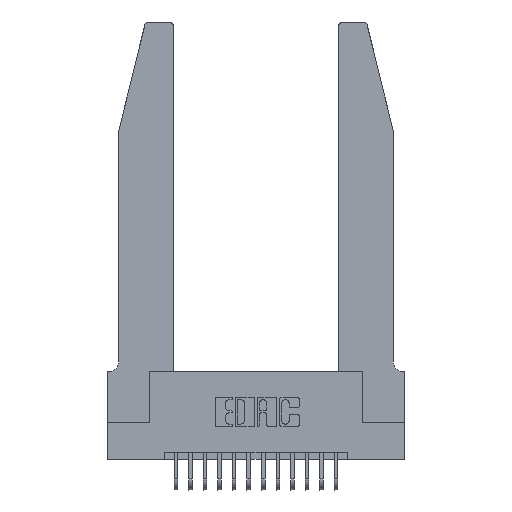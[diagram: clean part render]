
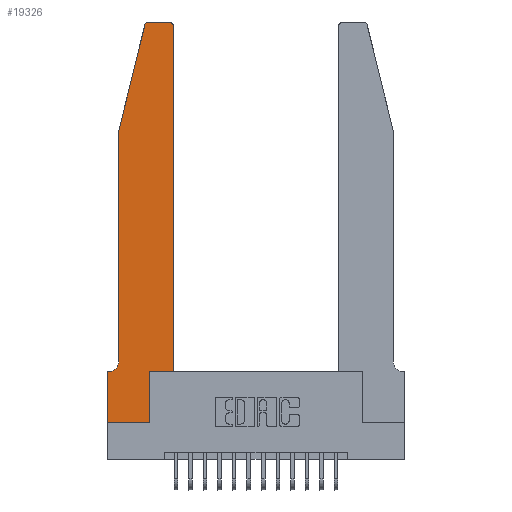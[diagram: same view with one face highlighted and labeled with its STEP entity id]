
A CAD part, top view. The second image highlights one B-rep face of the part: STEP entity #19326.
In plain terms, the highlighted planar face has unit normal (0, 0, 1).
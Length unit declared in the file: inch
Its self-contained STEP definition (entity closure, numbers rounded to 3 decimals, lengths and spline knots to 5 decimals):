
#26 = VERTEX_POINT ( 'NONE', #15186 ) ;
#244 = EDGE_CURVE ( 'NONE', #14576, #3467, #3808, .T. ) ;
#436 = LINE ( 'NONE', #11291, #12195 ) ;
#898 = VECTOR ( 'NONE', #17805, 39.37008 ) ;
#1098 = VECTOR ( 'NONE', #10412, 39.37008 ) ;
#1429 = VECTOR ( 'NONE', #11587, 39.37008 ) ;
#1484 = CARTESIAN_POINT ( 'NONE',  ( 0.0755, 2., 0.37 ) ) ;
#1569 = LINE ( 'NONE', #6275, #17394 ) ;
#1584 = CARTESIAN_POINT ( 'NONE',  ( 0.0755, 2., 0.37 ) ) ;
#1617 = EDGE_CURVE ( 'NONE', #3467, #6554, #19359, .T. ) ;
#2025 = VECTOR ( 'NONE', #5551, 39.37008 ) ;
#2248 = DIRECTION ( 'NONE',  ( 1., 0., 0. ) ) ;
#2370 = ORIENTED_EDGE ( 'NONE', *, *, #13172, .T. ) ;
#2454 = DIRECTION ( 'NONE',  ( 0., 0., 1. ) ) ;
#2817 = VERTEX_POINT ( 'NONE', #16610 ) ;
#2848 = EDGE_CURVE ( 'NONE', #11162, #7519, #9979, .T. ) ;
#3098 = ORIENTED_EDGE ( 'NONE', *, *, #8252, .T. ) ;
#3258 = ORIENTED_EDGE ( 'NONE', *, *, #15307, .T. ) ;
#3467 = VERTEX_POINT ( 'NONE', #10343 ) ;
#3624 = ORIENTED_EDGE ( 'NONE', *, *, #2848, .T. ) ;
#3808 = CIRCLE ( 'NONE', #12696, 0.03 ) ;
#4245 = AXIS2_PLACEMENT_3D ( 'NONE', #11985, #8992, #5958 ) ;
#4249 = EDGE_CURVE ( 'NONE', #6554, #26, #19289, .T. ) ;
#5144 = EDGE_CURVE ( 'NONE', #26, #11162, #10379, .T. ) ;
#5158 = CARTESIAN_POINT ( 'NONE',  ( 0., 0.35, 0.37 ) ) ;
#5329 = VERTEX_POINT ( 'NONE', #13268 ) ;
#5551 = DIRECTION ( 'NONE',  ( 0., 1., 0. ) ) ;
#5881 = ORIENTED_EDGE ( 'NONE', *, *, #18300, .T. ) ;
#5958 = DIRECTION ( 'NONE',  ( -1., 0., 0. ) ) ;
#6275 = CARTESIAN_POINT ( 'NONE',  ( 0., 0., 0.37 ) ) ;
#6293 = VECTOR ( 'NONE', #6874, 39.37008 ) ;
#6470 = LINE ( 'NONE', #18768, #8157 ) ;
#6519 = AXIS2_PLACEMENT_3D ( 'NONE', #12950, #2454, #14624 ) ;
#6554 = VERTEX_POINT ( 'NONE', #10840 ) ;
#6874 = DIRECTION ( 'NONE',  ( -0.239, -0.971, 0. ) ) ;
#7043 = ORIENTED_EDGE ( 'NONE', *, *, #8178, .T. ) ;
#7519 = VERTEX_POINT ( 'NONE', #9268 ) ;
#7778 = DIRECTION ( 'NONE',  ( 1., 0., 0. ) ) ;
#8123 = EDGE_LOOP ( 'NONE', ( #11698, #8226, #14193, #3624, #7043, #12957, #13219, #3098, #5881, #3258, #2370, #12021 ) ) ;
#8157 = VECTOR ( 'NONE', #18556, 39.37008 ) ;
#8178 = EDGE_CURVE ( 'NONE', #7519, #5329, #19112, .T. ) ;
#8226 = ORIENTED_EDGE ( 'NONE', *, *, #4249, .T. ) ;
#8252 = EDGE_CURVE ( 'NONE', #2817, #19585, #1569, .T. ) ;
#8663 = DIRECTION ( 'NONE',  ( 0., -1., 0. ) ) ;
#8667 = CARTESIAN_POINT ( 'NONE',  ( 0.2605, 2.75, 0.37 ) ) ;
#8739 = DIRECTION ( 'NONE',  ( 1., 0., 0. ) ) ;
#8992 = DIRECTION ( 'NONE',  ( 0., 0., -1. ) ) ;
#9268 = CARTESIAN_POINT ( 'NONE',  ( 0.0755, 0.42, 0.37 ) ) ;
#9979 = LINE ( 'NONE', #1484, #18391 ) ;
#10092 = CARTESIAN_POINT ( 'NONE',  ( 0.0755, 0.35, 0.37 ) ) ;
#10147 = FACE_OUTER_BOUND ( 'NONE', #8123, .T. ) ;
#10184 = LINE ( 'NONE', #14870, #2025 ) ;
#10224 = AXIS2_PLACEMENT_3D ( 'NONE', #16306, #10228, #8739 ) ;
#10228 = DIRECTION ( 'NONE',  ( 0., 0., 1. ) ) ;
#10343 = CARTESIAN_POINT ( 'NONE',  ( 0.4205, 2.75, 0.37 ) ) ;
#10379 = LINE ( 'NONE', #17712, #6293 ) ;
#10412 = DIRECTION ( 'NONE',  ( -1., 0., 0. ) ) ;
#10840 = CARTESIAN_POINT ( 'NONE',  ( 0.284, 2.75, 0.37 ) ) ;
#11162 = VERTEX_POINT ( 'NONE', #1584 ) ;
#11203 = VERTEX_POINT ( 'NONE', #18429 ) ;
#11219 = DIRECTION ( 'NONE',  ( 0., 1., 0. ) ) ;
#11252 = LINE ( 'NONE', #15246, #1429 ) ;
#11291 = CARTESIAN_POINT ( 'NONE',  ( 0.4505, 0.35, 0.37 ) ) ;
#11404 = DIRECTION ( 'NONE',  ( 0., 0., 1. ) ) ;
#11587 = DIRECTION ( 'NONE',  ( 0., -1., 0. ) ) ;
#11698 = ORIENTED_EDGE ( 'NONE', *, *, #1617, .T. ) ;
#11985 = CARTESIAN_POINT ( 'NONE',  ( 0.0055, 0.42, 0.37 ) ) ;
#12021 = ORIENTED_EDGE ( 'NONE', *, *, #244, .T. ) ;
#12188 = LINE ( 'NONE', #10092, #898 ) ;
#12195 = VECTOR ( 'NONE', #11219, 39.37008 ) ;
#12534 = VERTEX_POINT ( 'NONE', #15404 ) ;
#12584 = CARTESIAN_POINT ( 'NONE',  ( 0.4505, 2.72, 0.37 ) ) ;
#12696 = AXIS2_PLACEMENT_3D ( 'NONE', #17588, #11404, #2248 ) ;
#12950 = CARTESIAN_POINT ( 'NONE',  ( 0.284, 2.72, 0.37 ) ) ;
#12957 = ORIENTED_EDGE ( 'NONE', *, *, #15500, .T. ) ;
#13172 = EDGE_CURVE ( 'NONE', #11203, #14576, #436, .T. ) ;
#13218 = PLANE ( 'NONE',  #10224 ) ;
#13219 = ORIENTED_EDGE ( 'NONE', *, *, #14097, .T. ) ;
#13268 = CARTESIAN_POINT ( 'NONE',  ( 0.0055, 0.35, 0.37 ) ) ;
#14097 = EDGE_CURVE ( 'NONE', #16985, #2817, #11252, .T. ) ;
#14193 = ORIENTED_EDGE ( 'NONE', *, *, #5144, .T. ) ;
#14576 = VERTEX_POINT ( 'NONE', #12584 ) ;
#14624 = DIRECTION ( 'NONE',  ( 1., 0., 0. ) ) ;
#14870 = CARTESIAN_POINT ( 'NONE',  ( 0.2865, 0.35, 0.37 ) ) ;
#15186 = CARTESIAN_POINT ( 'NONE',  ( 0.25487, 2.72718, 0.37 ) ) ;
#15246 = CARTESIAN_POINT ( 'NONE',  ( 0., 0., 0.37 ) ) ;
#15307 = EDGE_CURVE ( 'NONE', #12534, #11203, #6470, .T. ) ;
#15404 = CARTESIAN_POINT ( 'NONE',  ( 0.2865, 0.35, 0.37 ) ) ;
#15500 = EDGE_CURVE ( 'NONE', #5329, #16985, #12188, .T. ) ;
#16306 = CARTESIAN_POINT ( 'NONE',  ( 0., 0.35, 0.37 ) ) ;
#16610 = CARTESIAN_POINT ( 'NONE',  ( 0., 0., 0.37 ) ) ;
#16985 = VERTEX_POINT ( 'NONE', #5158 ) ;
#17394 = VECTOR ( 'NONE', #7778, 39.37008 ) ;
#17588 = CARTESIAN_POINT ( 'NONE',  ( 0.4205, 2.72, 0.37 ) ) ;
#17712 = CARTESIAN_POINT ( 'NONE',  ( 0.0755, 2., 0.37 ) ) ;
#17805 = DIRECTION ( 'NONE',  ( -1., 0., 0. ) ) ;
#18300 = EDGE_CURVE ( 'NONE', #19585, #12534, #10184, .T. ) ;
#18391 = VECTOR ( 'NONE', #8663, 39.37008 ) ;
#18429 = CARTESIAN_POINT ( 'NONE',  ( 0.4505, 0.35, 0.37 ) ) ;
#18556 = DIRECTION ( 'NONE',  ( 1., 0., 0. ) ) ;
#18768 = CARTESIAN_POINT ( 'NONE',  ( 0.4505, 0.35, 0.37 ) ) ;
#19112 = CIRCLE ( 'NONE', #4245, 0.07 ) ;
#19289 = CIRCLE ( 'NONE', #6519, 0.03 ) ;
#19326 = ADVANCED_FACE ( 'NONE', ( #10147 ), #13218, .T. ) ;
#19359 = LINE ( 'NONE', #8667, #1098 ) ;
#19585 = VERTEX_POINT ( 'NONE', #19876 ) ;
#19876 = CARTESIAN_POINT ( 'NONE',  ( 0.2865, 0., 0.37 ) ) ;
